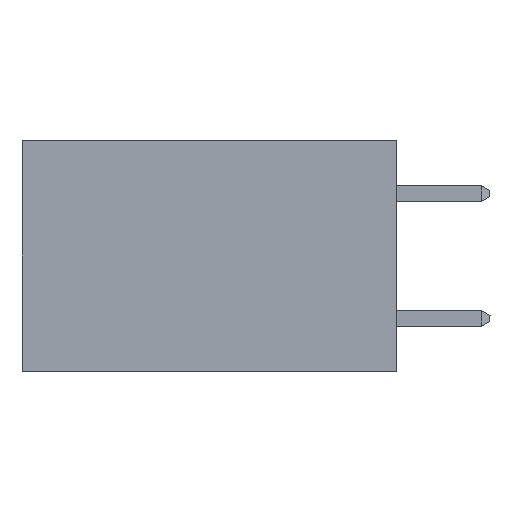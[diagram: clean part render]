
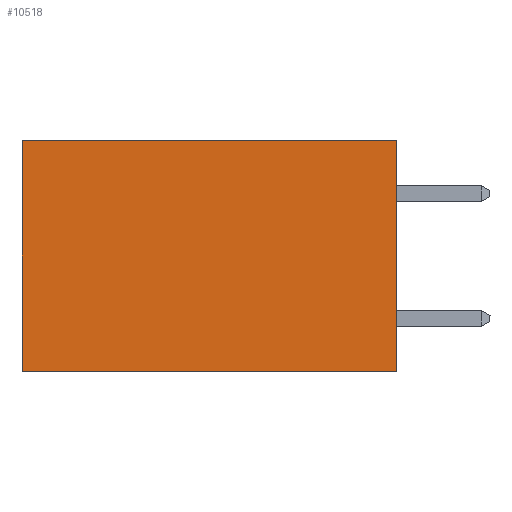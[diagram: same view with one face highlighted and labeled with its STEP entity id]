
A CAD part, left-side view. The second image highlights one B-rep face of the part: STEP entity #10518.
In plain terms, the highlighted planar face has unit normal (-1, 0, 0).
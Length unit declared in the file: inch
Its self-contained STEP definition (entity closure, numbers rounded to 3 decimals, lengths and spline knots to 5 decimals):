
#559 = VERTEX_POINT ( 'NONE', #7443 ) ;
#742 = CARTESIAN_POINT ( 'NONE',  ( 0.298, 0., -0.37 ) ) ;
#1552 = EDGE_CURVE ( 'NONE', #22732, #559, #3989, .T. ) ;
#2715 = CARTESIAN_POINT ( 'NONE',  ( 0.298, 0., 0. ) ) ;
#3006 = VECTOR ( 'NONE', #12839, 39.37008 ) ;
#3989 = LINE ( 'NONE', #15680, #27020 ) ;
#4404 = PLANE ( 'NONE',  #8653 ) ;
#5630 = EDGE_LOOP ( 'NONE', ( #14697, #9553, #18420, #8220 ) ) ;
#6697 = EDGE_CURVE ( 'NONE', #559, #25903, #16214, .T. ) ;
#7443 = CARTESIAN_POINT ( 'NONE',  ( 0.298, 0.6, 0. ) ) ;
#7604 = EDGE_CURVE ( 'NONE', #22732, #23432, #27453, .T. ) ;
#8220 = ORIENTED_EDGE ( 'NONE', *, *, #1552, .T. ) ;
#8653 = AXIS2_PLACEMENT_3D ( 'NONE', #20622, #22856, #9132 ) ;
#9132 = DIRECTION ( 'NONE',  ( 0., 0., -1. ) ) ;
#9553 = ORIENTED_EDGE ( 'NONE', *, *, #22072, .F. ) ;
#10518 = ADVANCED_FACE ( 'NONE', ( #20911 ), #4404, .F. ) ;
#12775 = CARTESIAN_POINT ( 'NONE',  ( 0.298, 0., -0.37 ) ) ;
#12839 = DIRECTION ( 'NONE',  ( 0., 0., -1. ) ) ;
#12864 = LINE ( 'NONE', #742, #17510 ) ;
#14697 = ORIENTED_EDGE ( 'NONE', *, *, #6697, .T. ) ;
#15680 = CARTESIAN_POINT ( 'NONE',  ( 0.298, 0., 0. ) ) ;
#16126 = DIRECTION ( 'NONE',  ( 0., 0., -1. ) ) ;
#16214 = LINE ( 'NONE', #16565, #27509 ) ;
#16565 = CARTESIAN_POINT ( 'NONE',  ( 0.298, 0.6, 0. ) ) ;
#16909 = CARTESIAN_POINT ( 'NONE',  ( 0.298, 0., 0. ) ) ;
#17510 = VECTOR ( 'NONE', #19311, 39.37008 ) ;
#18420 = ORIENTED_EDGE ( 'NONE', *, *, #7604, .F. ) ;
#19311 = DIRECTION ( 'NONE',  ( 0., 1., 0. ) ) ;
#20622 = CARTESIAN_POINT ( 'NONE',  ( 0.298, 0., 0. ) ) ;
#20911 = FACE_OUTER_BOUND ( 'NONE', #5630, .T. ) ;
#22072 = EDGE_CURVE ( 'NONE', #23432, #25903, #12864, .T. ) ;
#22732 = VERTEX_POINT ( 'NONE', #16909 ) ;
#22856 = DIRECTION ( 'NONE',  ( 1., 0., 0. ) ) ;
#23143 = DIRECTION ( 'NONE',  ( 0., 1., 0. ) ) ;
#23432 = VERTEX_POINT ( 'NONE', #12775 ) ;
#25903 = VERTEX_POINT ( 'NONE', #26751 ) ;
#26751 = CARTESIAN_POINT ( 'NONE',  ( 0.298, 0.6, -0.37 ) ) ;
#27020 = VECTOR ( 'NONE', #23143, 39.37008 ) ;
#27453 = LINE ( 'NONE', #2715, #3006 ) ;
#27509 = VECTOR ( 'NONE', #16126, 39.37008 ) ;
